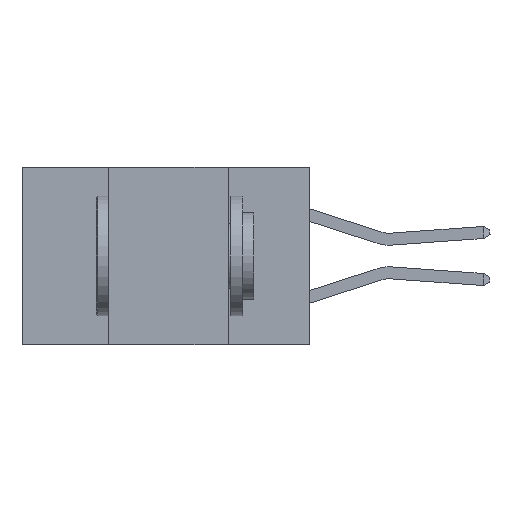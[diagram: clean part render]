
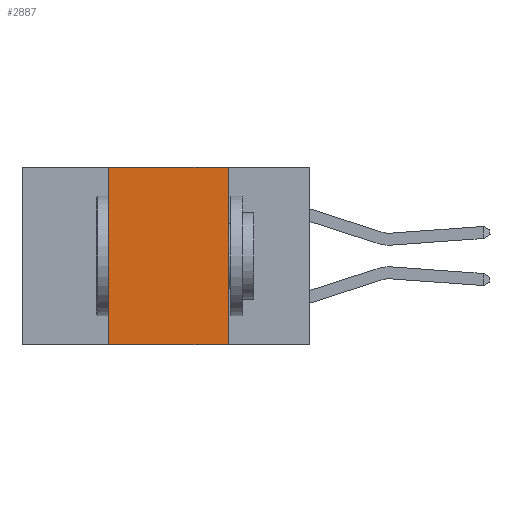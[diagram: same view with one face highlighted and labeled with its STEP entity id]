
A CAD part, left-side view. The second image highlights one B-rep face of the part: STEP entity #2887.
In plain terms, the highlighted planar face has unit normal (-1, 0, 0).
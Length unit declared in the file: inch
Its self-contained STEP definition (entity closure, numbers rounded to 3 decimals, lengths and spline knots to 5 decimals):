
#206 = LINE ( 'NONE', #8500, #8827 ) ;
#311 = VECTOR ( 'NONE', #4104, 39.37008 ) ;
#539 = CARTESIAN_POINT ( 'NONE',  ( 0., 0.17, -0.37 ) ) ;
#687 = DIRECTION ( 'NONE',  ( 0., -1., 0. ) ) ;
#1585 = VECTOR ( 'NONE', #687, 39.37008 ) ;
#1678 = AXIS2_PLACEMENT_3D ( 'NONE', #2236, #2348, #2315 ) ;
#2236 = CARTESIAN_POINT ( 'NONE',  ( 0., 0.6, 0. ) ) ;
#2271 = PLANE ( 'NONE',  #1678 ) ;
#2315 = DIRECTION ( 'NONE',  ( 0., 0., -1. ) ) ;
#2348 = DIRECTION ( 'NONE',  ( 1., 0., 0. ) ) ;
#2390 = FACE_OUTER_BOUND ( 'NONE', #5571, .T. ) ;
#2874 = ORIENTED_EDGE ( 'NONE', *, *, #4260, .F. ) ;
#2887 = ADVANCED_FACE ( 'NONE', ( #2390 ), #2271, .F. ) ;
#3999 = CARTESIAN_POINT ( 'NONE',  ( 0., 0.17, 0. ) ) ;
#4104 = DIRECTION ( 'NONE',  ( 0., 0., -1. ) ) ;
#4132 = CARTESIAN_POINT ( 'NONE',  ( 0., 0.17, 0. ) ) ;
#4165 = CARTESIAN_POINT ( 'NONE',  ( 0., 0.42, -0.37 ) ) ;
#4260 = EDGE_CURVE ( 'NONE', #6972, #5453, #206, .T. ) ;
#4419 = ORIENTED_EDGE ( 'NONE', *, *, #5021, .F. ) ;
#4772 = CARTESIAN_POINT ( 'NONE',  ( 0., 0.42, 0. ) ) ;
#4843 = VERTEX_POINT ( 'NONE', #539 ) ;
#4993 = LINE ( 'NONE', #8386, #9352 ) ;
#5021 = EDGE_CURVE ( 'NONE', #5453, #4843, #6864, .T. ) ;
#5060 = ORIENTED_EDGE ( 'NONE', *, *, #6712, .F. ) ;
#5453 = VERTEX_POINT ( 'NONE', #4132 ) ;
#5571 = EDGE_LOOP ( 'NONE', ( #4419, #2874, #5060, #9542 ) ) ;
#5580 = EDGE_CURVE ( 'NONE', #6302, #4843, #8098, .T. ) ;
#6302 = VERTEX_POINT ( 'NONE', #4165 ) ;
#6712 = EDGE_CURVE ( 'NONE', #6302, #6972, #4993, .T. ) ;
#6725 = CARTESIAN_POINT ( 'NONE',  ( 0., 0.6, -0.37 ) ) ;
#6864 = LINE ( 'NONE', #3999, #311 ) ;
#6972 = VERTEX_POINT ( 'NONE', #4772 ) ;
#7787 = DIRECTION ( 'NONE',  ( 0., -1., 0. ) ) ;
#8098 = LINE ( 'NONE', #6725, #1585 ) ;
#8386 = CARTESIAN_POINT ( 'NONE',  ( 0., 0.42, 0. ) ) ;
#8500 = CARTESIAN_POINT ( 'NONE',  ( 0., 0.6, 0. ) ) ;
#8827 = VECTOR ( 'NONE', #7787, 39.37008 ) ;
#9352 = VECTOR ( 'NONE', #9523, 39.37008 ) ;
#9523 = DIRECTION ( 'NONE',  ( 0., 0., 1. ) ) ;
#9542 = ORIENTED_EDGE ( 'NONE', *, *, #5580, .T. ) ;
